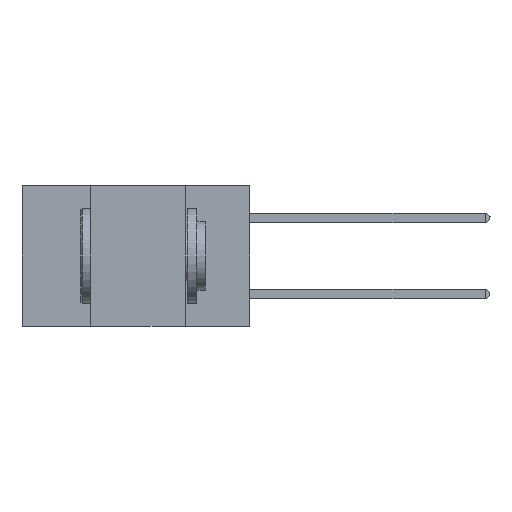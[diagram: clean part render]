
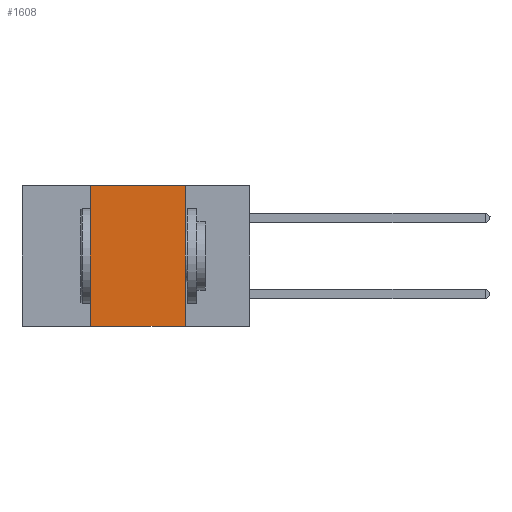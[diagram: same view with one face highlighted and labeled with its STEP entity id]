
A CAD part, left-side view. The second image highlights one B-rep face of the part: STEP entity #1608.
In plain terms, the highlighted planar face has unit normal (-1, 0, 0).
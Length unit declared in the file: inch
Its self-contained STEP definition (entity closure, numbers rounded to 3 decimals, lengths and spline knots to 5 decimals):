
#94 = DIRECTION ( 'NONE',  ( 0., -1., 0. ) ) ;
#289 = EDGE_CURVE ( 'NONE', #7931, #8792, #9431, .T. ) ;
#1386 = VERTEX_POINT ( 'NONE', #2310 ) ;
#1575 = AXIS2_PLACEMENT_3D ( 'NONE', #4563, #4544, #4524 ) ;
#1608 = ADVANCED_FACE ( 'NONE', ( #9151 ), #4826, .F. ) ;
#1895 = LINE ( 'NONE', #3666, #7074 ) ;
#2310 = CARTESIAN_POINT ( 'NONE',  ( 0., 0.17, -0.37 ) ) ;
#3146 = LINE ( 'NONE', #8644, #7896 ) ;
#3168 = ORIENTED_EDGE ( 'NONE', *, *, #289, .F. ) ;
#3666 = CARTESIAN_POINT ( 'NONE',  ( 0., 0.42, 0. ) ) ;
#3823 = LINE ( 'NONE', #4521, #6386 ) ;
#4521 = CARTESIAN_POINT ( 'NONE',  ( 0., 0.6, -0.37 ) ) ;
#4524 = DIRECTION ( 'NONE',  ( 0., 0., -1. ) ) ;
#4539 = DIRECTION ( 'NONE',  ( 0., -1., 0. ) ) ;
#4544 = DIRECTION ( 'NONE',  ( 1., 0., 0. ) ) ;
#4563 = CARTESIAN_POINT ( 'NONE',  ( 0., 0.6, 0. ) ) ;
#4635 = EDGE_LOOP ( 'NONE', ( #4953, #3168, #9826, #7724 ) ) ;
#4826 = PLANE ( 'NONE',  #1575 ) ;
#4923 = DIRECTION ( 'NONE',  ( 0., 0., -1. ) ) ;
#4953 = ORIENTED_EDGE ( 'NONE', *, *, #7950, .F. ) ;
#5480 = EDGE_CURVE ( 'NONE', #11999, #1386, #3823, .T. ) ;
#6341 = CARTESIAN_POINT ( 'NONE',  ( 0., 0.42, -0.37 ) ) ;
#6386 = VECTOR ( 'NONE', #4539, 39.37008 ) ;
#7046 = VECTOR ( 'NONE', #94, 39.37008 ) ;
#7074 = VECTOR ( 'NONE', #7427, 39.37008 ) ;
#7427 = DIRECTION ( 'NONE',  ( 0., 0., 1. ) ) ;
#7724 = ORIENTED_EDGE ( 'NONE', *, *, #5480, .T. ) ;
#7896 = VECTOR ( 'NONE', #4923, 39.37008 ) ;
#7931 = VERTEX_POINT ( 'NONE', #9504 ) ;
#7950 = EDGE_CURVE ( 'NONE', #8792, #1386, #3146, .T. ) ;
#8644 = CARTESIAN_POINT ( 'NONE',  ( 0., 0.17, 0. ) ) ;
#8792 = VERTEX_POINT ( 'NONE', #9212 ) ;
#9151 = FACE_OUTER_BOUND ( 'NONE', #4635, .T. ) ;
#9212 = CARTESIAN_POINT ( 'NONE',  ( 0., 0.17, 0. ) ) ;
#9431 = LINE ( 'NONE', #11138, #7046 ) ;
#9504 = CARTESIAN_POINT ( 'NONE',  ( 0., 0.42, 0. ) ) ;
#9826 = ORIENTED_EDGE ( 'NONE', *, *, #12108, .F. ) ;
#11138 = CARTESIAN_POINT ( 'NONE',  ( 0., 0.6, 0. ) ) ;
#11999 = VERTEX_POINT ( 'NONE', #6341 ) ;
#12108 = EDGE_CURVE ( 'NONE', #11999, #7931, #1895, .T. ) ;
